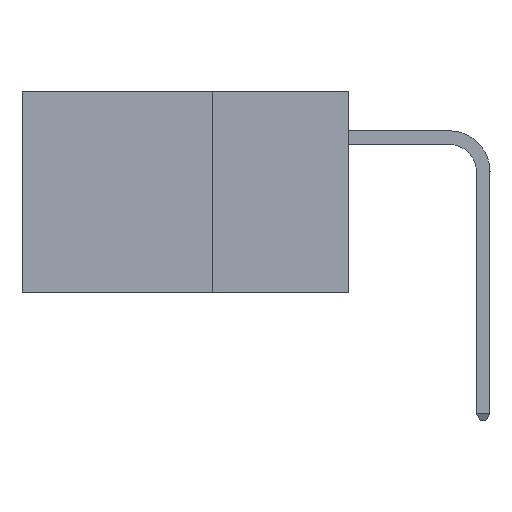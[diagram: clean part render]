
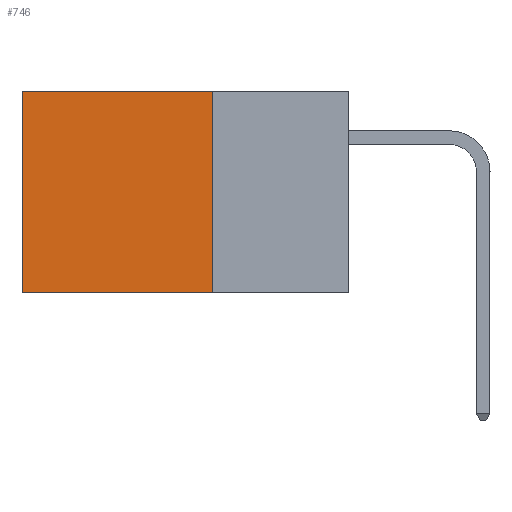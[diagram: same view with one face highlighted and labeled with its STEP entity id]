
A CAD part, left-side view. The second image highlights one B-rep face of the part: STEP entity #746.
In plain terms, the highlighted planar face has unit normal (-1, 0, 0).
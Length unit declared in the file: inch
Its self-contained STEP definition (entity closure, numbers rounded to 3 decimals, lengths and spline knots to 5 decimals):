
#292 = EDGE_CURVE ( 'NONE', #6505, #12775, #9184, .T. ) ;
#458 = VECTOR ( 'NONE', #13175, 39.37008 ) ;
#593 = ORIENTED_EDGE ( 'NONE', *, *, #11978, .T. ) ;
#746 = ADVANCED_FACE ( 'NONE', ( #5248 ), #3289, .F. ) ;
#912 = VECTOR ( 'NONE', #12969, 39.37008 ) ;
#1100 = CARTESIAN_POINT ( 'NONE',  ( 0.2875, 0.25, 0. ) ) ;
#1252 = CARTESIAN_POINT ( 'NONE',  ( 0.2875, 0.25, 0. ) ) ;
#2114 = ORIENTED_EDGE ( 'NONE', *, *, #292, .F. ) ;
#2962 = CARTESIAN_POINT ( 'NONE',  ( 0.2875, 0.6, 0. ) ) ;
#2978 = EDGE_CURVE ( 'NONE', #16049, #6505, #3991, .T. ) ;
#3141 = VERTEX_POINT ( 'NONE', #2962 ) ;
#3204 = DIRECTION ( 'NONE',  ( 0., 1., 0. ) ) ;
#3286 = CARTESIAN_POINT ( 'NONE',  ( 0.2875, 0.25, 0. ) ) ;
#3289 = PLANE ( 'NONE',  #5418 ) ;
#3576 = CARTESIAN_POINT ( 'NONE',  ( 0.2875, 0.25, -0.37 ) ) ;
#3991 = LINE ( 'NONE', #1252, #912 ) ;
#4205 = DIRECTION ( 'NONE',  ( 0., 1., 0. ) ) ;
#4908 = ORIENTED_EDGE ( 'NONE', *, *, #2978, .F. ) ;
#5248 = FACE_OUTER_BOUND ( 'NONE', #7765, .T. ) ;
#5418 = AXIS2_PLACEMENT_3D ( 'NONE', #3286, #5622, #5758 ) ;
#5622 = DIRECTION ( 'NONE',  ( 1., 0., 0. ) ) ;
#5758 = DIRECTION ( 'NONE',  ( 0., 0., -1. ) ) ;
#5946 = CARTESIAN_POINT ( 'NONE',  ( 0.2875, 0.6, -0.37 ) ) ;
#6505 = VERTEX_POINT ( 'NONE', #11270 ) ;
#7765 = EDGE_LOOP ( 'NONE', ( #593, #2114, #4908, #13609 ) ) ;
#7898 = VECTOR ( 'NONE', #3204, 39.37008 ) ;
#9184 = LINE ( 'NONE', #3576, #12171 ) ;
#10932 = LINE ( 'NONE', #14462, #458 ) ;
#11034 = CARTESIAN_POINT ( 'NONE',  ( 0.2875, 0.25, 0. ) ) ;
#11270 = CARTESIAN_POINT ( 'NONE',  ( 0.2875, 0.25, -0.37 ) ) ;
#11538 = EDGE_CURVE ( 'NONE', #16049, #3141, #11736, .T. ) ;
#11736 = LINE ( 'NONE', #11034, #7898 ) ;
#11978 = EDGE_CURVE ( 'NONE', #3141, #12775, #10932, .T. ) ;
#12171 = VECTOR ( 'NONE', #4205, 39.37008 ) ;
#12775 = VERTEX_POINT ( 'NONE', #5946 ) ;
#12969 = DIRECTION ( 'NONE',  ( 0., 0., -1. ) ) ;
#13175 = DIRECTION ( 'NONE',  ( 0., 0., -1. ) ) ;
#13609 = ORIENTED_EDGE ( 'NONE', *, *, #11538, .T. ) ;
#14462 = CARTESIAN_POINT ( 'NONE',  ( 0.2875, 0.6, 0. ) ) ;
#16049 = VERTEX_POINT ( 'NONE', #1100 ) ;
